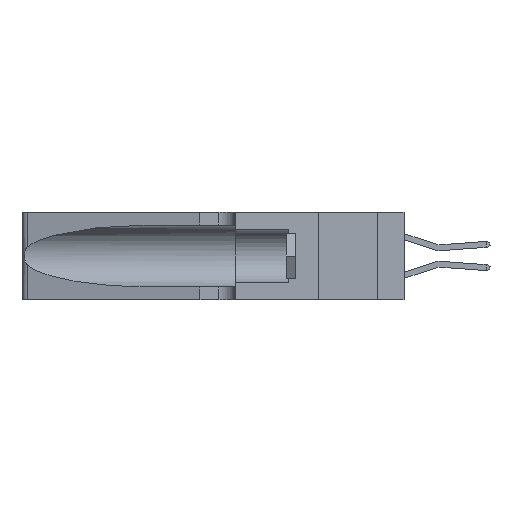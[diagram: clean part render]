
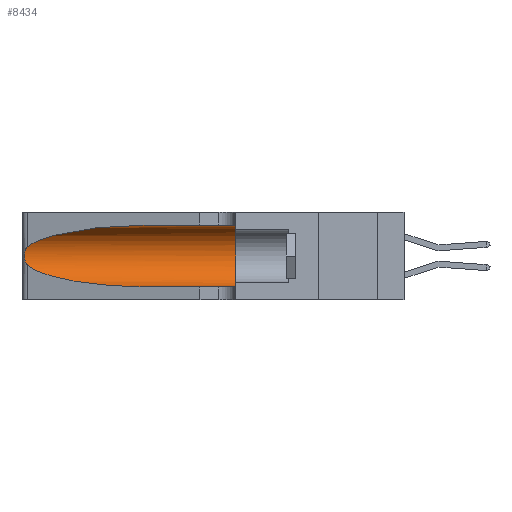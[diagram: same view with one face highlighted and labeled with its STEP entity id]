
A CAD part, left-side view. The second image highlights one B-rep face of the part: STEP entity #8434.
In plain terms, the highlighted cylindrical face has radius 3.308 mm (diameter 6.617 mm), a partial arc.
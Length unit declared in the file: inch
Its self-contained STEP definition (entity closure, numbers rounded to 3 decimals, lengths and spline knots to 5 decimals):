
#14 = EDGE_CURVE ( 'NONE', #19082, #22863, #4582, .T. ) ;
#124 = DIRECTION ( 'NONE',  ( 0., -1., 0. ) ) ;
#150 =( BOUNDED_CURVE ( )  B_SPLINE_CURVE ( 3, ( #16338, #4899, #6579, #2902 ),
 .UNSPECIFIED., .F., .F. ) 
 B_SPLINE_CURVE_WITH_KNOTS ( ( 4, 4 ),
 ( 3.44316, 4.71239 ),
 .UNSPECIFIED. ) 
 CURVE ( )  GEOMETRIC_REPRESENTATION_ITEM ( )  RATIONAL_B_SPLINE_CURVE ( ( 1., 0.87, 0.87, 1. ) ) 
 REPRESENTATION_ITEM ( '' )  );
#554 = CYLINDRICAL_SURFACE ( 'NONE', #5378, 0.13025 ) ;
#848 = CARTESIAN_POINT ( 'NONE',  ( 0.25639, 1.23186, 0.15144 ) ) ;
#1965 = EDGE_LOOP ( 'NONE', ( #11296, #21139, #10132, #11194, #22886, #15273 ) ) ;
#2462 = CARTESIAN_POINT ( 'NONE',  ( 0.25487, 1.22718, 0.22369 ) ) ;
#2688 = CARTESIAN_POINT ( 'NONE',  ( 0.26075, 1.23896, 0.178 ) ) ;
#2902 = CARTESIAN_POINT ( 'NONE',  ( 0.1305, 0.72297, 0.05475 ) ) ;
#4182 = EDGE_CURVE ( 'NONE', #22767, #10309, #150, .T. ) ;
#4582 =( BOUNDED_CURVE ( )  B_SPLINE_CURVE ( 3, ( #10200, #6288, #21936, #10378 ),
 .UNSPECIFIED., .F., .F. ) 
 B_SPLINE_CURVE_WITH_KNOTS ( ( 4, 4 ),
 ( 1.5708, 2.84003 ),
 .UNSPECIFIED. ) 
 CURVE ( )  GEOMETRIC_REPRESENTATION_ITEM ( )  RATIONAL_B_SPLINE_CURVE ( ( 1., 0.87, 0.87, 1. ) ) 
 REPRESENTATION_ITEM ( '' )  );
#4899 = CARTESIAN_POINT ( 'NONE',  ( 0.2373, 1.15595, 0.08982 ) ) ;
#4934 = CARTESIAN_POINT ( 'NONE',  ( 0.25555, 1.22994, 0.2215 ) ) ;
#5378 = AXIS2_PLACEMENT_3D ( 'NONE', #9049, #7196, #24592 ) ;
#6288 = CARTESIAN_POINT ( 'NONE',  ( 0.18966, 0.96281, 0.31525 ) ) ;
#6527 = CARTESIAN_POINT ( 'NONE',  ( 0.26017, 1.23833, 0.17102 ) ) ;
#6579 = CARTESIAN_POINT ( 'NONE',  ( 0.18966, 0.96281, 0.05475 ) ) ;
#7124 = EDGE_CURVE ( 'NONE', #22863, #22767, #8029, .T. ) ;
#7196 = DIRECTION ( 'NONE',  ( 0., -1., 0. ) ) ;
#7580 = CARTESIAN_POINT ( 'NONE',  ( 0.1305, 1.61858, 0.05475 ) ) ;
#7691 = DIRECTION ( 'NONE',  ( 0., 1., 0. ) ) ;
#7709 = FACE_OUTER_BOUND ( 'NONE', #1965, .T. ) ;
#7943 = EDGE_CURVE ( 'NONE', #10309, #17323, #16841, .T. ) ;
#7947 = VECTOR ( 'NONE', #19342, 39.37008 ) ;
#8029 = B_SPLINE_CURVE_WITH_KNOTS ( 'NONE', 3,
 ( #20245, #4934, #20407, #16291, #18198, #10772, #14246, #2688, #6527, #21997, #23931, #848, #20163, #8546 ),
 .UNSPECIFIED., .F., .F.,
 ( 4, 2, 2, 2, 2, 2, 4 ),
 ( 0., 0.00027, 0.00053, 0.00107, 0.0016, 0.00187, 0.00214 ),
 .UNSPECIFIED. ) ;
#8434 = ADVANCED_FACE ( 'NONE', ( #7709 ), #554, .F. ) ;
#8546 = CARTESIAN_POINT ( 'NONE',  ( 0.25487, 1.22718, 0.14631 ) ) ;
#9049 = CARTESIAN_POINT ( 'NONE',  ( 0.1305, 1.61858, 0.185 ) ) ;
#9220 = CARTESIAN_POINT ( 'NONE',  ( 0.1305, 0.72297, 0.31525 ) ) ;
#9742 = CARTESIAN_POINT ( 'NONE',  ( 0.1305, 0.35, 0.31525 ) ) ;
#10073 = CARTESIAN_POINT ( 'NONE',  ( 0.1305, 0.72297, 0.05475 ) ) ;
#10132 = ORIENTED_EDGE ( 'NONE', *, *, #4182, .T. ) ;
#10200 = CARTESIAN_POINT ( 'NONE',  ( 0.1305, 0.72297, 0.31525 ) ) ;
#10309 = VERTEX_POINT ( 'NONE', #10073 ) ;
#10378 = CARTESIAN_POINT ( 'NONE',  ( 0.25487, 1.22718, 0.22369 ) ) ;
#10772 = CARTESIAN_POINT ( 'NONE',  ( 0.26018, 1.23835, 0.19895 ) ) ;
#11194 = ORIENTED_EDGE ( 'NONE', *, *, #7943, .T. ) ;
#11296 = ORIENTED_EDGE ( 'NONE', *, *, #14, .T. ) ;
#11624 = CARTESIAN_POINT ( 'NONE',  ( 0.1305, 0.35, 0.185 ) ) ;
#13504 = VECTOR ( 'NONE', #124, 39.37008 ) ;
#14246 = CARTESIAN_POINT ( 'NONE',  ( 0.26075, 1.23896, 0.19203 ) ) ;
#14376 = EDGE_CURVE ( 'NONE', #19082, #24790, #24861, .T. ) ;
#15273 = ORIENTED_EDGE ( 'NONE', *, *, #14376, .F. ) ;
#15430 = DIRECTION ( 'NONE',  ( 0., 0., 1. ) ) ;
#15495 = AXIS2_PLACEMENT_3D ( 'NONE', #11624, #7691, #15430 ) ;
#16291 = CARTESIAN_POINT ( 'NONE',  ( 0.25787, 1.23484, 0.2124 ) ) ;
#16338 = CARTESIAN_POINT ( 'NONE',  ( 0.25487, 1.22718, 0.14631 ) ) ;
#16841 = LINE ( 'NONE', #7580, #13504 ) ;
#17323 = VERTEX_POINT ( 'NONE', #19850 ) ;
#17403 = CARTESIAN_POINT ( 'NONE',  ( 0.1305, 1.61858, 0.31525 ) ) ;
#18198 = CARTESIAN_POINT ( 'NONE',  ( 0.25854, 1.2359, 0.20912 ) ) ;
#19082 = VERTEX_POINT ( 'NONE', #9220 ) ;
#19342 = DIRECTION ( 'NONE',  ( 0., -1., 0. ) ) ;
#19850 = CARTESIAN_POINT ( 'NONE',  ( 0.1305, 0.35, 0.05475 ) ) ;
#20163 = CARTESIAN_POINT ( 'NONE',  ( 0.25555, 1.22993, 0.14849 ) ) ;
#20245 = CARTESIAN_POINT ( 'NONE',  ( 0.25487, 1.22718, 0.22369 ) ) ;
#20407 = CARTESIAN_POINT ( 'NONE',  ( 0.25639, 1.23184, 0.21858 ) ) ;
#20894 = CIRCLE ( 'NONE', #15495, 0.13025 ) ;
#21139 = ORIENTED_EDGE ( 'NONE', *, *, #7124, .T. ) ;
#21936 = CARTESIAN_POINT ( 'NONE',  ( 0.2373, 1.15595, 0.28018 ) ) ;
#21997 = CARTESIAN_POINT ( 'NONE',  ( 0.25856, 1.23593, 0.16098 ) ) ;
#22767 = VERTEX_POINT ( 'NONE', #23591 ) ;
#22863 = VERTEX_POINT ( 'NONE', #2462 ) ;
#22886 = ORIENTED_EDGE ( 'NONE', *, *, #23021, .F. ) ;
#23021 = EDGE_CURVE ( 'NONE', #24790, #17323, #20894, .T. ) ;
#23591 = CARTESIAN_POINT ( 'NONE',  ( 0.25487, 1.22718, 0.14631 ) ) ;
#23931 = CARTESIAN_POINT ( 'NONE',  ( 0.25789, 1.23486, 0.15765 ) ) ;
#24592 = DIRECTION ( 'NONE',  ( 0., 0., -1. ) ) ;
#24790 = VERTEX_POINT ( 'NONE', #9742 ) ;
#24861 = LINE ( 'NONE', #17403, #7947 ) ;
